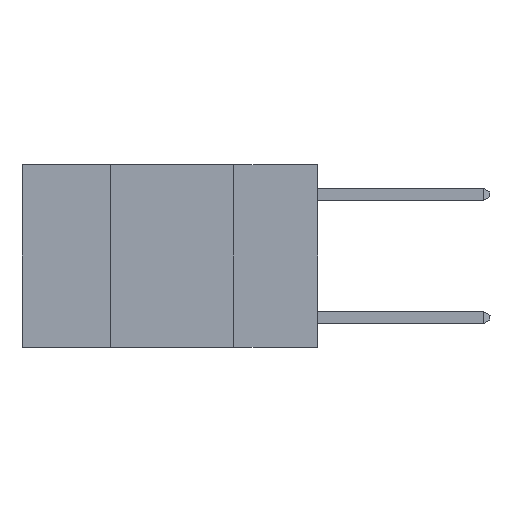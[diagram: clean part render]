
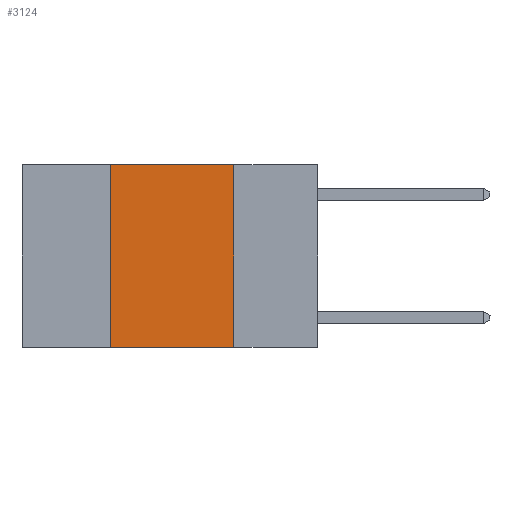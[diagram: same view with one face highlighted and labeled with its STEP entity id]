
A CAD part, left-side view. The second image highlights one B-rep face of the part: STEP entity #3124.
In plain terms, the highlighted planar face has unit normal (-1, 0, 0).
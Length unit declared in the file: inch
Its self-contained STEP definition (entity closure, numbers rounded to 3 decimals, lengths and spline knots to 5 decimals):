
#82 = LINE ( 'NONE', #4795, #8478 ) ;
#169 = EDGE_CURVE ( 'NONE', #5705, #627, #82, .T. ) ;
#245 = EDGE_CURVE ( 'NONE', #8761, #8814, #2283, .T. ) ;
#493 = PLANE ( 'NONE',  #10919 ) ;
#531 = CARTESIAN_POINT ( 'NONE',  ( 0., 0.6, 0. ) ) ;
#627 = VERTEX_POINT ( 'NONE', #7377 ) ;
#777 = EDGE_LOOP ( 'NONE', ( #6156, #6012, #5045, #11053 ) ) ;
#885 = LINE ( 'NONE', #531, #3212 ) ;
#1103 = DIRECTION ( 'NONE',  ( 0., 0., -1. ) ) ;
#1584 = DIRECTION ( 'NONE',  ( 1., 0., 0. ) ) ;
#1738 = CARTESIAN_POINT ( 'NONE',  ( 0., 0.42, -0.37 ) ) ;
#2283 = LINE ( 'NONE', #11040, #10125 ) ;
#3124 = ADVANCED_FACE ( 'NONE', ( #10309 ), #493, .F. ) ;
#3212 = VECTOR ( 'NONE', #8922, 39.37008 ) ;
#4795 = CARTESIAN_POINT ( 'NONE',  ( 0., 0.17, 0. ) ) ;
#4877 = CARTESIAN_POINT ( 'NONE',  ( 0., 0.6, 0. ) ) ;
#5015 = VECTOR ( 'NONE', #11865, 39.37008 ) ;
#5045 = ORIENTED_EDGE ( 'NONE', *, *, #245, .F. ) ;
#5705 = VERTEX_POINT ( 'NONE', #5932 ) ;
#5932 = CARTESIAN_POINT ( 'NONE',  ( 0., 0.17, 0. ) ) ;
#6012 = ORIENTED_EDGE ( 'NONE', *, *, #13060, .F. ) ;
#6156 = ORIENTED_EDGE ( 'NONE', *, *, #169, .F. ) ;
#7076 = CARTESIAN_POINT ( 'NONE',  ( 0., 0.42, 0. ) ) ;
#7377 = CARTESIAN_POINT ( 'NONE',  ( 0., 0.17, -0.37 ) ) ;
#7588 = EDGE_CURVE ( 'NONE', #8761, #627, #7705, .T. ) ;
#7705 = LINE ( 'NONE', #9022, #5015 ) ;
#8478 = VECTOR ( 'NONE', #1103, 39.37008 ) ;
#8761 = VERTEX_POINT ( 'NONE', #1738 ) ;
#8814 = VERTEX_POINT ( 'NONE', #7076 ) ;
#8889 = DIRECTION ( 'NONE',  ( 0., 0., -1. ) ) ;
#8922 = DIRECTION ( 'NONE',  ( 0., -1., 0. ) ) ;
#9022 = CARTESIAN_POINT ( 'NONE',  ( 0., 0.6, -0.37 ) ) ;
#10125 = VECTOR ( 'NONE', #11334, 39.37008 ) ;
#10309 = FACE_OUTER_BOUND ( 'NONE', #777, .T. ) ;
#10919 = AXIS2_PLACEMENT_3D ( 'NONE', #4877, #1584, #8889 ) ;
#11040 = CARTESIAN_POINT ( 'NONE',  ( 0., 0.42, 0. ) ) ;
#11053 = ORIENTED_EDGE ( 'NONE', *, *, #7588, .T. ) ;
#11334 = DIRECTION ( 'NONE',  ( 0., 0., 1. ) ) ;
#11865 = DIRECTION ( 'NONE',  ( 0., -1., 0. ) ) ;
#13060 = EDGE_CURVE ( 'NONE', #8814, #5705, #885, .T. ) ;
